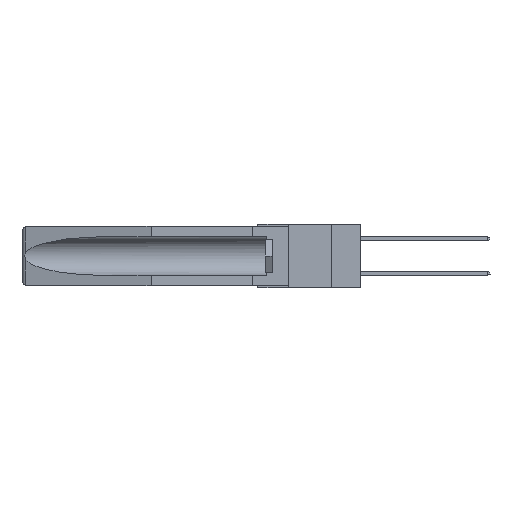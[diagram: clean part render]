
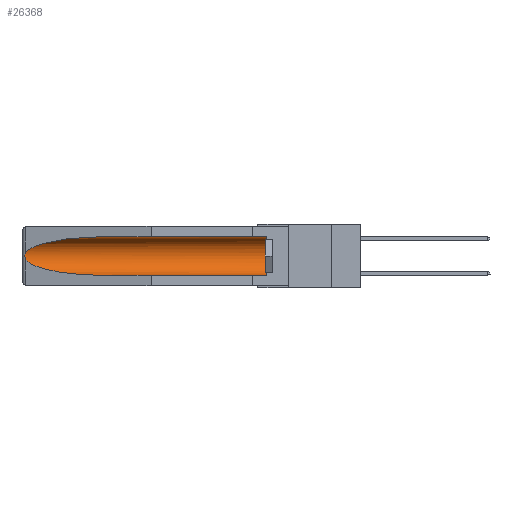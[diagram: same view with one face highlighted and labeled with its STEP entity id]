
A CAD part, left-side view. The second image highlights one B-rep face of the part: STEP entity #26368.
In plain terms, the highlighted cylindrical face has radius 2.857 mm (diameter 5.715 mm), a partial arc.
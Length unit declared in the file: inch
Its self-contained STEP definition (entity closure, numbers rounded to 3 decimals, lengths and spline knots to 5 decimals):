
#41 = CARTESIAN_POINT ( 'NONE',  ( 0.26655, 1.53094, -0.18657 ) ) ;
#365 = EDGE_CURVE ( 'NONE', #8817, #10007, #29276, .T. ) ;
#402 = CARTESIAN_POINT ( 'NONE',  ( 0.26537, 1.52718, -0.19328 ) ) ;
#507 = CARTESIAN_POINT ( 'NONE',  ( 0.155, 1.07973, -0.284 ) ) ;
#1526 =( BOUNDED_CURVE ( )  B_SPLINE_CURVE ( 3, ( #11671, #22424, #25151, #27372 ),
 .UNSPECIFIED., .F., .F. ) 
 B_SPLINE_CURVE_WITH_KNOTS ( ( 4, 4 ),
 ( 4.71239, 6.08839 ),
 .UNSPECIFIED. ) 
 CURVE ( )  GEOMETRIC_REPRESENTATION_ITEM ( )  RATIONAL_B_SPLINE_CURVE ( ( 1., 0.848, 0.848, 1. ) ) 
 REPRESENTATION_ITEM ( '' )  );
#1751 = CARTESIAN_POINT ( 'NONE',  ( 0.26537, 1.52718, -0.19328 ) ) ;
#2355 = CARTESIAN_POINT ( 'NONE',  ( 0.155, -0.30754, -0.059 ) ) ;
#2567 = CARTESIAN_POINT ( 'NONE',  ( 0.2675, 1.53308, -0.16763 ) ) ;
#2594 = EDGE_CURVE ( 'NONE', #10007, #7309, #1526, .T. ) ;
#2919 = ORIENTED_EDGE ( 'NONE', *, *, #18427, .T. ) ;
#3413 = EDGE_LOOP ( 'NONE', ( #32056, #22321, #2919, #26465, #4089, #7152 ) ) ;
#3508 = CARTESIAN_POINT ( 'NONE',  ( 0.155, -0.30754, -0.284 ) ) ;
#4089 = ORIENTED_EDGE ( 'NONE', *, *, #27436, .T. ) ;
#5115 = FACE_OUTER_BOUND ( 'NONE', #3413, .T. ) ;
#5769 = CARTESIAN_POINT ( 'NONE',  ( 0.155, 1.07973, -0.059 ) ) ;
#6259 = DIRECTION ( 'NONE',  ( 0., 0., 1. ) ) ;
#6352 = CARTESIAN_POINT ( 'NONE',  ( 0.155, 0.126, -0.284 ) ) ;
#7152 = ORIENTED_EDGE ( 'NONE', *, *, #365, .T. ) ;
#7309 = VERTEX_POINT ( 'NONE', #18141 ) ;
#7604 = EDGE_CURVE ( 'NONE', #7309, #7860, #10666, .T. ) ;
#7803 = CARTESIAN_POINT ( 'NONE',  ( 0.2675, 1.53308, -0.17534 ) ) ;
#7860 = VERTEX_POINT ( 'NONE', #12103 ) ;
#8684 = CIRCLE ( 'NONE', #26754, 0.1125 ) ;
#8817 = VERTEX_POINT ( 'NONE', #30293 ) ;
#10007 = VERTEX_POINT ( 'NONE', #5769 ) ;
#10278 = CARTESIAN_POINT ( 'NONE',  ( 0.26537, 1.52718, -0.14972 ) ) ;
#10666 = B_SPLINE_CURVE_WITH_KNOTS ( 'NONE', 3,
 ( #10278, #28471, #28258, #18082, #2567, #7803, #31211, #41, #33032, #1751 ),
 .UNSPECIFIED., .F., .F.,
 ( 4, 2, 2, 2, 4 ),
 ( 0., 0.00029, 0.00058, 0.00087, 0.00117 ),
 .UNSPECIFIED. ) ;
#11436 = VERTEX_POINT ( 'NONE', #6352 ) ;
#11671 = CARTESIAN_POINT ( 'NONE',  ( 0.155, 1.07973, -0.059 ) ) ;
#11790 = CARTESIAN_POINT ( 'NONE',  ( 0.155, -0.30754, -0.1715 ) ) ;
#12103 = CARTESIAN_POINT ( 'NONE',  ( 0.26537, 1.52718, -0.19328 ) ) ;
#16052 = CARTESIAN_POINT ( 'NONE',  ( 0.21114, 1.30732, -0.284 ) ) ;
#16789 = DIRECTION ( 'NONE',  ( 0., 1., 0. ) ) ;
#18082 = CARTESIAN_POINT ( 'NONE',  ( 0.2673, 1.5327, -0.16383 ) ) ;
#18141 = CARTESIAN_POINT ( 'NONE',  ( 0.26537, 1.52718, -0.14972 ) ) ;
#18226 = VERTEX_POINT ( 'NONE', #25731 ) ;
#18427 = EDGE_CURVE ( 'NONE', #7860, #18226, #20310, .T. ) ;
#18584 = CARTESIAN_POINT ( 'NONE',  ( 0.25451, 1.48313, -0.24835 ) ) ;
#20310 =( BOUNDED_CURVE ( )  B_SPLINE_CURVE ( 3, ( #402, #18584, #16052, #507 ),
 .UNSPECIFIED., .F., .F. ) 
 B_SPLINE_CURVE_WITH_KNOTS ( ( 4, 4 ),
 ( 0.1948, 1.5708 ),
 .UNSPECIFIED. ) 
 CURVE ( )  GEOMETRIC_REPRESENTATION_ITEM ( )  RATIONAL_B_SPLINE_CURVE ( ( 1., 0.848, 0.848, 1. ) ) 
 REPRESENTATION_ITEM ( '' )  );
#21497 = AXIS2_PLACEMENT_3D ( 'NONE', #11790, #16789, #6259 ) ;
#21625 = VECTOR ( 'NONE', #21699, 39.37008 ) ;
#21699 = DIRECTION ( 'NONE',  ( 0., 1., 0. ) ) ;
#21867 = DIRECTION ( 'NONE',  ( 0., -1., 0. ) ) ;
#22321 = ORIENTED_EDGE ( 'NONE', *, *, #7604, .T. ) ;
#22424 = CARTESIAN_POINT ( 'NONE',  ( 0.21114, 1.30732, -0.059 ) ) ;
#23070 = DIRECTION ( 'NONE',  ( 0., 1., 0. ) ) ;
#25151 = CARTESIAN_POINT ( 'NONE',  ( 0.25451, 1.48313, -0.09465 ) ) ;
#25731 = CARTESIAN_POINT ( 'NONE',  ( 0.155, 1.07973, -0.284 ) ) ;
#26368 = ADVANCED_FACE ( 'NONE', ( #5115 ), #33174, .F. ) ;
#26465 = ORIENTED_EDGE ( 'NONE', *, *, #31601, .F. ) ;
#26617 = DIRECTION ( 'NONE',  ( 0., 0., 1. ) ) ;
#26754 = AXIS2_PLACEMENT_3D ( 'NONE', #31864, #21867, #26617 ) ;
#27372 = CARTESIAN_POINT ( 'NONE',  ( 0.26537, 1.52718, -0.14972 ) ) ;
#27436 = EDGE_CURVE ( 'NONE', #11436, #8817, #8684, .T. ) ;
#28258 = CARTESIAN_POINT ( 'NONE',  ( 0.26654, 1.53092, -0.15636 ) ) ;
#28471 = CARTESIAN_POINT ( 'NONE',  ( 0.26597, 1.52961, -0.15275 ) ) ;
#29276 = LINE ( 'NONE', #2355, #30111 ) ;
#29320 = LINE ( 'NONE', #3508, #21625 ) ;
#30111 = VECTOR ( 'NONE', #23070, 39.37008 ) ;
#30293 = CARTESIAN_POINT ( 'NONE',  ( 0.155, 0.126, -0.059 ) ) ;
#31211 = CARTESIAN_POINT ( 'NONE',  ( 0.2673, 1.53269, -0.17917 ) ) ;
#31601 = EDGE_CURVE ( 'NONE', #11436, #18226, #29320, .T. ) ;
#31864 = CARTESIAN_POINT ( 'NONE',  ( 0.155, 0.126, -0.1715 ) ) ;
#32056 = ORIENTED_EDGE ( 'NONE', *, *, #2594, .T. ) ;
#33032 = CARTESIAN_POINT ( 'NONE',  ( 0.26597, 1.5296, -0.19026 ) ) ;
#33174 = CYLINDRICAL_SURFACE ( 'NONE', #21497, 0.1125 ) ;
